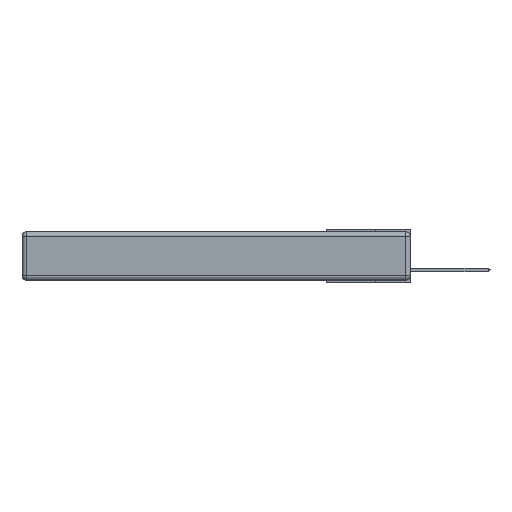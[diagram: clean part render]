
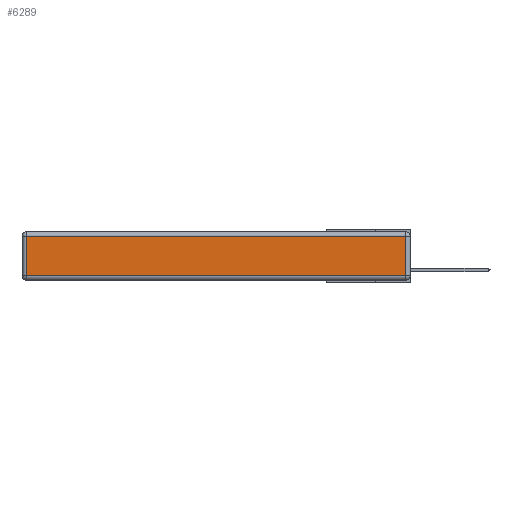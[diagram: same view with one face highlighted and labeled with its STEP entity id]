
A CAD part, left-side view. The second image highlights one B-rep face of the part: STEP entity #6289.
In plain terms, the highlighted planar face has unit normal (-1, 0, 0).
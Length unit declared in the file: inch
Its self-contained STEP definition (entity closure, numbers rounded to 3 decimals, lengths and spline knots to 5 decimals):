
#1092 = DIRECTION ( 'NONE',  ( -1., 0., 0. ) ) ;
#1567 = CARTESIAN_POINT ( 'NONE',  ( 0., 2.72, -0.313 ) ) ;
#3460 = DIRECTION ( 'NONE',  ( 0., 0., 1. ) ) ;
#4705 = CARTESIAN_POINT ( 'NONE',  ( 0., 2.72, -0.03 ) ) ;
#5352 = EDGE_CURVE ( 'NONE', #15184, #11002, #16358, .T. ) ;
#5945 = VECTOR ( 'NONE', #21579, 39.37008 ) ;
#6215 = LINE ( 'NONE', #21922, #17629 ) ;
#6289 = ADVANCED_FACE ( 'NONE', ( #11331 ), #30285, .T. ) ;
#6458 = VERTEX_POINT ( 'NONE', #4705 ) ;
#8113 = EDGE_CURVE ( 'NONE', #6458, #15184, #11963, .T. ) ;
#8229 = EDGE_LOOP ( 'NONE', ( #29810, #16270, #28611, #19050 ) ) ;
#9171 = EDGE_CURVE ( 'NONE', #18703, #6458, #6215, .T. ) ;
#9655 = DIRECTION ( 'NONE',  ( 0., 1., 0. ) ) ;
#9730 = LINE ( 'NONE', #31554, #30754 ) ;
#11002 = VERTEX_POINT ( 'NONE', #28055 ) ;
#11331 = FACE_OUTER_BOUND ( 'NONE', #8229, .T. ) ;
#11963 = LINE ( 'NONE', #23632, #5945 ) ;
#12355 = DIRECTION ( 'NONE',  ( 0., 0., 1. ) ) ;
#15184 = VERTEX_POINT ( 'NONE', #1567 ) ;
#16270 = ORIENTED_EDGE ( 'NONE', *, *, #26953, .T. ) ;
#16358 = LINE ( 'NONE', #25795, #27082 ) ;
#17629 = VECTOR ( 'NONE', #9655, 39.37008 ) ;
#18535 = DIRECTION ( 'NONE',  ( 0., -1., 0. ) ) ;
#18703 = VERTEX_POINT ( 'NONE', #27948 ) ;
#19050 = ORIENTED_EDGE ( 'NONE', *, *, #8113, .T. ) ;
#21579 = DIRECTION ( 'NONE',  ( 0., 0., -1. ) ) ;
#21922 = CARTESIAN_POINT ( 'NONE',  ( 0., 2.75, -0.03 ) ) ;
#22805 = CARTESIAN_POINT ( 'NONE',  ( 0., 0., -0.343 ) ) ;
#23632 = CARTESIAN_POINT ( 'NONE',  ( 0., 2.72, -0.343 ) ) ;
#24529 = AXIS2_PLACEMENT_3D ( 'NONE', #22805, #1092, #3460 ) ;
#25795 = CARTESIAN_POINT ( 'NONE',  ( 0., 0., -0.313 ) ) ;
#26953 = EDGE_CURVE ( 'NONE', #11002, #18703, #9730, .T. ) ;
#27082 = VECTOR ( 'NONE', #18535, 39.37008 ) ;
#27948 = CARTESIAN_POINT ( 'NONE',  ( 0., 0.03, -0.03 ) ) ;
#28055 = CARTESIAN_POINT ( 'NONE',  ( 0., 0.03, -0.313 ) ) ;
#28611 = ORIENTED_EDGE ( 'NONE', *, *, #9171, .T. ) ;
#29810 = ORIENTED_EDGE ( 'NONE', *, *, #5352, .T. ) ;
#30285 = PLANE ( 'NONE',  #24529 ) ;
#30754 = VECTOR ( 'NONE', #12355, 39.37008 ) ;
#31554 = CARTESIAN_POINT ( 'NONE',  ( 0., 0.03, -0.343 ) ) ;
